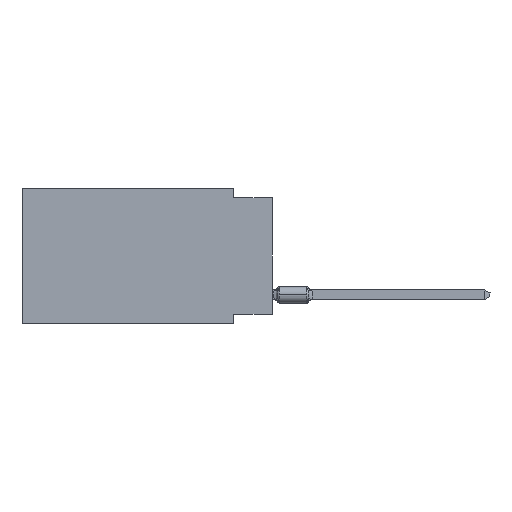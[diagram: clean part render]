
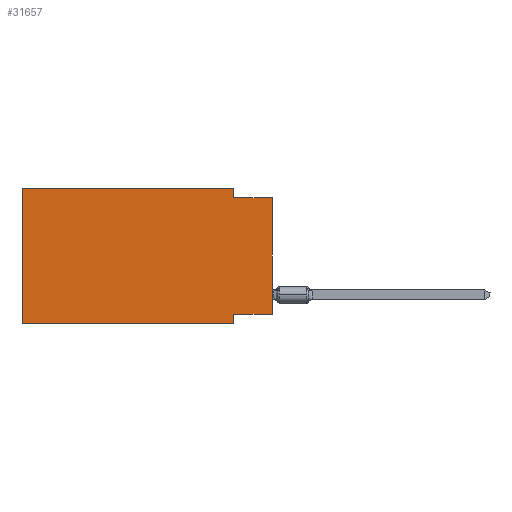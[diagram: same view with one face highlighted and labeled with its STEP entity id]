
A CAD part, left-side view. The second image highlights one B-rep face of the part: STEP entity #31657.
In plain terms, the highlighted planar face has unit normal (-1, 0, 0).
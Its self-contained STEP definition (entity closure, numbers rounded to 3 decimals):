
#55 = LINE ( 'NONE', #10580, #12481 ) ;
#915 = CARTESIAN_POINT ( 'NONE',  ( 0., 16.383, 0. ) ) ;
#1641 = CARTESIAN_POINT ( 'NONE',  ( 0., 16.383, 0. ) ) ;
#3060 = EDGE_CURVE ( 'NONE', #31929, #21428, #25097, .T. ) ;
#3752 = VECTOR ( 'NONE', #10553, 1000. ) ;
#4350 = CARTESIAN_POINT ( 'NONE',  ( 0., 16.383, -8.89 ) ) ;
#4531 = CARTESIAN_POINT ( 'NONE',  ( 0., 16.383, -8.89 ) ) ;
#5245 = CARTESIAN_POINT ( 'NONE',  ( 0., 2.54, -8.89 ) ) ;
#5959 = DIRECTION ( 'NONE',  ( 0., 0., -1. ) ) ;
#6339 = EDGE_CURVE ( 'NONE', #16276, #16820, #35424, .T. ) ;
#6431 = DIRECTION ( 'NONE',  ( 0., 0., 1. ) ) ;
#7147 = DIRECTION ( 'NONE',  ( 0., 0., -1. ) ) ;
#7776 = LINE ( 'NONE', #915, #11815 ) ;
#8605 = VECTOR ( 'NONE', #10837, 1000. ) ;
#9854 = CARTESIAN_POINT ( 'NONE',  ( 0., 16.383, 0. ) ) ;
#9869 = ORIENTED_EDGE ( 'NONE', *, *, #30236, .F. ) ;
#9926 = LINE ( 'NONE', #17004, #8605 ) ;
#10553 = DIRECTION ( 'NONE',  ( 0., 1., 0. ) ) ;
#10580 = CARTESIAN_POINT ( 'NONE',  ( 0., 2.54, -8.89 ) ) ;
#10837 = DIRECTION ( 'NONE',  ( 0., 0., 1. ) ) ;
#11815 = VECTOR ( 'NONE', #21033, 1000. ) ;
#12481 = VECTOR ( 'NONE', #7147, 1000. ) ;
#12691 = CARTESIAN_POINT ( 'NONE',  ( 0., 0., -8.255 ) ) ;
#15291 = DIRECTION ( 'NONE',  ( 0., -1., 0. ) ) ;
#15378 = ORIENTED_EDGE ( 'NONE', *, *, #44199, .F. ) ;
#15562 = AXIS2_PLACEMENT_3D ( 'NONE', #9854, #16714, #5959 ) ;
#15623 = VERTEX_POINT ( 'NONE', #28983 ) ;
#15633 = ORIENTED_EDGE ( 'NONE', *, *, #39849, .F. ) ;
#16276 = VERTEX_POINT ( 'NONE', #35477 ) ;
#16372 = DIRECTION ( 'NONE',  ( 0., -1., 0. ) ) ;
#16714 = DIRECTION ( 'NONE',  ( 1., 0., 0. ) ) ;
#16820 = VERTEX_POINT ( 'NONE', #24365 ) ;
#16971 = ORIENTED_EDGE ( 'NONE', *, *, #26675, .F. ) ;
#17004 = CARTESIAN_POINT ( 'NONE',  ( 0., 16.383, 0. ) ) ;
#18110 = CARTESIAN_POINT ( 'NONE',  ( 0., 2.54, 0. ) ) ;
#20131 = LINE ( 'NONE', #30627, #3752 ) ;
#20137 = LINE ( 'NONE', #34266, #29061 ) ;
#20653 = CARTESIAN_POINT ( 'NONE',  ( 0., 2.54, -8.255 ) ) ;
#20684 = VERTEX_POINT ( 'NONE', #20653 ) ;
#21033 = DIRECTION ( 'NONE',  ( 0., -1., 0. ) ) ;
#21428 = VERTEX_POINT ( 'NONE', #5245 ) ;
#22404 = VECTOR ( 'NONE', #28599, 1000. ) ;
#22417 = VECTOR ( 'NONE', #16372, 1000. ) ;
#22888 = ORIENTED_EDGE ( 'NONE', *, *, #3060, .T. ) ;
#23431 = LINE ( 'NONE', #27304, #22417 ) ;
#24365 = CARTESIAN_POINT ( 'NONE',  ( 0., 2.54, -0.635 ) ) ;
#24899 = VERTEX_POINT ( 'NONE', #12691 ) ;
#25097 = LINE ( 'NONE', #4531, #32376 ) ;
#26675 = EDGE_CURVE ( 'NONE', #31929, #40558, #9926, .T. ) ;
#27240 = EDGE_CURVE ( 'NONE', #24899, #15623, #20137, .T. ) ;
#27304 = CARTESIAN_POINT ( 'NONE',  ( 0., 0., -0.635 ) ) ;
#28599 = DIRECTION ( 'NONE',  ( 0., 0., -1. ) ) ;
#28879 = ORIENTED_EDGE ( 'NONE', *, *, #6339, .F. ) ;
#28983 = CARTESIAN_POINT ( 'NONE',  ( 0., 0., -0.635 ) ) ;
#29061 = VECTOR ( 'NONE', #6431, 1000. ) ;
#29404 = EDGE_CURVE ( 'NONE', #24899, #20684, #20131, .T. ) ;
#29510 = ORIENTED_EDGE ( 'NONE', *, *, #27240, .T. ) ;
#30236 = EDGE_CURVE ( 'NONE', #40558, #16276, #7776, .T. ) ;
#30627 = CARTESIAN_POINT ( 'NONE',  ( 0., 0., -8.255 ) ) ;
#31657 = ADVANCED_FACE ( 'NONE', ( #33807 ), #37015, .F. ) ;
#31929 = VERTEX_POINT ( 'NONE', #4350 ) ;
#32376 = VECTOR ( 'NONE', #15291, 1000. ) ;
#33807 = FACE_OUTER_BOUND ( 'NONE', #41264, .T. ) ;
#34252 = ORIENTED_EDGE ( 'NONE', *, *, #29404, .F. ) ;
#34266 = CARTESIAN_POINT ( 'NONE',  ( 0., 0., 0. ) ) ;
#35424 = LINE ( 'NONE', #18110, #22404 ) ;
#35477 = CARTESIAN_POINT ( 'NONE',  ( 0., 2.54, 0. ) ) ;
#37015 = PLANE ( 'NONE',  #15562 ) ;
#39849 = EDGE_CURVE ( 'NONE', #16820, #15623, #23431, .T. ) ;
#40558 = VERTEX_POINT ( 'NONE', #1641 ) ;
#41264 = EDGE_LOOP ( 'NONE', ( #29510, #15633, #28879, #9869, #16971, #22888, #15378, #34252 ) ) ;
#44199 = EDGE_CURVE ( 'NONE', #20684, #21428, #55, .T. ) ;
